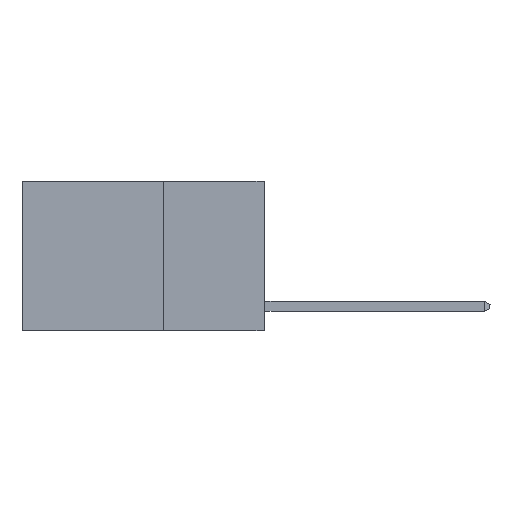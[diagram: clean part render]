
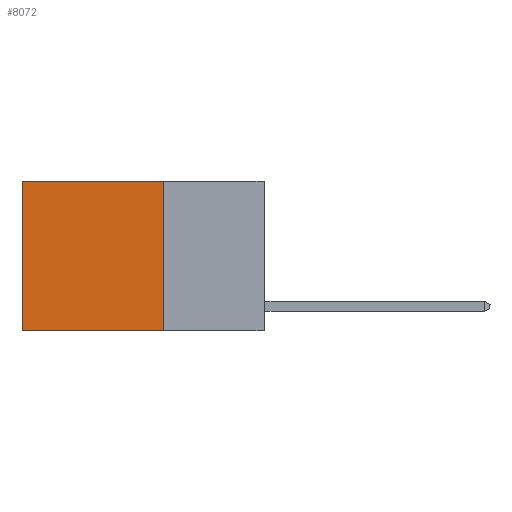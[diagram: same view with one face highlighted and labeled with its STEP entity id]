
A CAD part, left-side view. The second image highlights one B-rep face of the part: STEP entity #8072.
In plain terms, the highlighted planar face has unit normal (-1, 0, 0).
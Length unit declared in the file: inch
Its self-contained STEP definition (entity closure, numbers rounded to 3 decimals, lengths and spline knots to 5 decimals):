
#293 = CARTESIAN_POINT ( 'NONE',  ( 0.2625, 0.25, 0. ) ) ;
#633 = ORIENTED_EDGE ( 'NONE', *, *, #3633, .T. ) ;
#827 = CARTESIAN_POINT ( 'NONE',  ( 0.2625, 0.6, 0. ) ) ;
#893 = DIRECTION ( 'NONE',  ( 0., 1., 0. ) ) ;
#946 = LINE ( 'NONE', #4452, #5729 ) ;
#1342 = VERTEX_POINT ( 'NONE', #827 ) ;
#1390 = VECTOR ( 'NONE', #6978, 39.37008 ) ;
#1728 = CARTESIAN_POINT ( 'NONE',  ( 0.2625, 0.6, 0. ) ) ;
#1858 = AXIS2_PLACEMENT_3D ( 'NONE', #11660, #3289, #9835 ) ;
#1972 = VECTOR ( 'NONE', #893, 39.37008 ) ;
#3289 = DIRECTION ( 'NONE',  ( 1., 0., 0. ) ) ;
#3376 = EDGE_CURVE ( 'NONE', #1342, #6686, #3750, .T. ) ;
#3512 = DIRECTION ( 'NONE',  ( 0., 0., -1. ) ) ;
#3633 = EDGE_CURVE ( 'NONE', #8738, #1342, #10820, .T. ) ;
#3750 = LINE ( 'NONE', #1728, #11193 ) ;
#3834 = EDGE_CURVE ( 'NONE', #8738, #8155, #946, .T. ) ;
#4010 = EDGE_CURVE ( 'NONE', #8155, #6686, #11393, .T. ) ;
#4135 = CARTESIAN_POINT ( 'NONE',  ( 0.2625, 0.25, 0. ) ) ;
#4310 = CARTESIAN_POINT ( 'NONE',  ( 0.2625, 0.25, -0.37 ) ) ;
#4452 = CARTESIAN_POINT ( 'NONE',  ( 0.2625, 0.25, 0. ) ) ;
#5542 = ORIENTED_EDGE ( 'NONE', *, *, #3376, .T. ) ;
#5729 = VECTOR ( 'NONE', #3512, 39.37008 ) ;
#6686 = VERTEX_POINT ( 'NONE', #12149 ) ;
#6978 = DIRECTION ( 'NONE',  ( 0., 1., 0. ) ) ;
#7388 = FACE_OUTER_BOUND ( 'NONE', #8975, .T. ) ;
#7550 = CARTESIAN_POINT ( 'NONE',  ( 0.2625, 0.25, -0.37 ) ) ;
#7968 = ORIENTED_EDGE ( 'NONE', *, *, #3834, .F. ) ;
#8072 = ADVANCED_FACE ( 'NONE', ( #7388 ), #8914, .F. ) ;
#8155 = VERTEX_POINT ( 'NONE', #4310 ) ;
#8738 = VERTEX_POINT ( 'NONE', #4135 ) ;
#8914 = PLANE ( 'NONE',  #1858 ) ;
#8975 = EDGE_LOOP ( 'NONE', ( #5542, #11095, #7968, #633 ) ) ;
#9291 = DIRECTION ( 'NONE',  ( 0., 0., -1. ) ) ;
#9835 = DIRECTION ( 'NONE',  ( 0., 0., -1. ) ) ;
#10820 = LINE ( 'NONE', #293, #1390 ) ;
#11095 = ORIENTED_EDGE ( 'NONE', *, *, #4010, .F. ) ;
#11193 = VECTOR ( 'NONE', #9291, 39.37008 ) ;
#11393 = LINE ( 'NONE', #7550, #1972 ) ;
#11660 = CARTESIAN_POINT ( 'NONE',  ( 0.2625, 0.25, 0. ) ) ;
#12149 = CARTESIAN_POINT ( 'NONE',  ( 0.2625, 0.6, -0.37 ) ) ;
